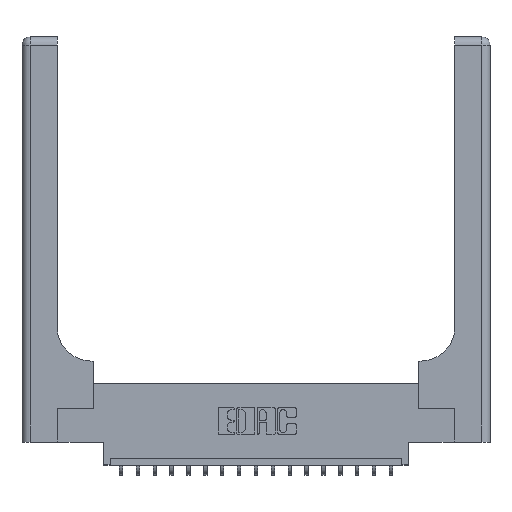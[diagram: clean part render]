
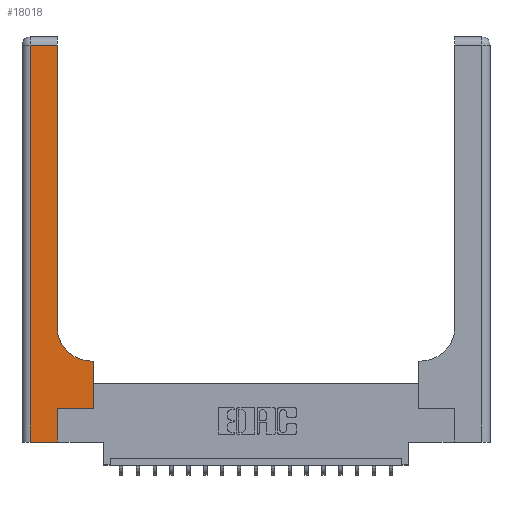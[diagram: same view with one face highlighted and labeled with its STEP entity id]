
A CAD part, top view. The second image highlights one B-rep face of the part: STEP entity #18018.
In plain terms, the highlighted planar face has unit normal (0, 0, 1).
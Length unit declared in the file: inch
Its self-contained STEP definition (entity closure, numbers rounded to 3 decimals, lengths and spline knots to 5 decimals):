
#52 = EDGE_CURVE ( 'NONE', #16930, #7713, #11292, .T. ) ;
#722 = EDGE_LOOP ( 'NONE', ( #4917, #16883, #13863, #2828, #6843, #11314, #15719, #741, #4698 ) ) ;
#741 = ORIENTED_EDGE ( 'NONE', *, *, #16131, .T. ) ;
#763 = VERTEX_POINT ( 'NONE', #7768 ) ;
#984 = DIRECTION ( 'NONE',  ( 1., 0., 0. ) ) ;
#1055 = EDGE_CURVE ( 'NONE', #16804, #16004, #9851, .T. ) ;
#1430 = VERTEX_POINT ( 'NONE', #13749 ) ;
#1799 = CARTESIAN_POINT ( 'NONE',  ( 0.26, 0.85, 0.37 ) ) ;
#2469 = CARTESIAN_POINT ( 'NONE',  ( 0.26, 2.94, 0.37 ) ) ;
#2828 = ORIENTED_EDGE ( 'NONE', *, *, #13575, .T. ) ;
#3823 = LINE ( 'NONE', #15802, #11369 ) ;
#4076 = DIRECTION ( 'NONE',  ( 0., 1., 0. ) ) ;
#4698 = ORIENTED_EDGE ( 'NONE', *, *, #8506, .T. ) ;
#4772 = PLANE ( 'NONE',  #10855 ) ;
#4830 = VERTEX_POINT ( 'NONE', #11650 ) ;
#4917 = ORIENTED_EDGE ( 'NONE', *, *, #7274, .T. ) ;
#5082 = VERTEX_POINT ( 'NONE', #1799 ) ;
#5216 = LINE ( 'NONE', #12580, #8334 ) ;
#5824 = VECTOR ( 'NONE', #984, 39.37008 ) ;
#5890 = VECTOR ( 'NONE', #4076, 39.37008 ) ;
#6302 = CARTESIAN_POINT ( 'NONE',  ( 0., 3., 0.37 ) ) ;
#6549 = CARTESIAN_POINT ( 'NONE',  ( 0.51, 0.85, 0.37 ) ) ;
#6659 = DIRECTION ( 'NONE',  ( -1., 0., 0. ) ) ;
#6843 = ORIENTED_EDGE ( 'NONE', *, *, #10674, .T. ) ;
#6967 = AXIS2_PLACEMENT_3D ( 'NONE', #6549, #16999, #8089 ) ;
#7274 = EDGE_CURVE ( 'NONE', #5082, #8728, #3823, .T. ) ;
#7713 = VERTEX_POINT ( 'NONE', #15285 ) ;
#7768 = CARTESIAN_POINT ( 'NONE',  ( 0.265, 0., 0.37 ) ) ;
#7836 = DIRECTION ( 'NONE',  ( 0., 0., -1. ) ) ;
#8089 = DIRECTION ( 'NONE',  ( 1., 0., 0. ) ) ;
#8334 = VECTOR ( 'NONE', #11222, 39.37008 ) ;
#8506 = EDGE_CURVE ( 'NONE', #1430, #5082, #15771, .T. ) ;
#8728 = VERTEX_POINT ( 'NONE', #2469 ) ;
#9010 = CARTESIAN_POINT ( 'NONE',  ( 0.528, 0.25, 0.37 ) ) ;
#9616 = FACE_OUTER_BOUND ( 'NONE', #722, .T. ) ;
#9851 = LINE ( 'NONE', #18771, #5824 ) ;
#10055 = DIRECTION ( 'NONE',  ( 1., 0., 0. ) ) ;
#10365 = VECTOR ( 'NONE', #19259, 39.37008 ) ;
#10436 = CARTESIAN_POINT ( 'NONE',  ( 0.06, 3., 0.37 ) ) ;
#10502 = DIRECTION ( 'NONE',  ( 0., 1., 0. ) ) ;
#10674 = EDGE_CURVE ( 'NONE', #763, #16804, #19159, .T. ) ;
#10782 = EDGE_CURVE ( 'NONE', #16004, #4830, #12474, .T. ) ;
#10855 = AXIS2_PLACEMENT_3D ( 'NONE', #6302, #7836, #18221 ) ;
#11222 = DIRECTION ( 'NONE',  ( -1., 0., 0. ) ) ;
#11264 = CARTESIAN_POINT ( 'NONE',  ( 0.265, 0.25, 0.37 ) ) ;
#11292 = LINE ( 'NONE', #10436, #10365 ) ;
#11314 = ORIENTED_EDGE ( 'NONE', *, *, #1055, .T. ) ;
#11369 = VECTOR ( 'NONE', #17298, 39.37008 ) ;
#11650 = CARTESIAN_POINT ( 'NONE',  ( 0.528, 0.6, 0.37 ) ) ;
#12358 = VECTOR ( 'NONE', #10055, 39.37008 ) ;
#12474 = LINE ( 'NONE', #9010, #15951 ) ;
#12580 = CARTESIAN_POINT ( 'NONE',  ( 0.26, 0.6, 0.37 ) ) ;
#13575 = EDGE_CURVE ( 'NONE', #7713, #763, #16302, .T. ) ;
#13690 = CARTESIAN_POINT ( 'NONE',  ( 0.528, 0.25, 0.37 ) ) ;
#13749 = CARTESIAN_POINT ( 'NONE',  ( 0.51, 0.6, 0.37 ) ) ;
#13863 = ORIENTED_EDGE ( 'NONE', *, *, #52, .T. ) ;
#14120 = EDGE_CURVE ( 'NONE', #8728, #16930, #18785, .T. ) ;
#14462 = CARTESIAN_POINT ( 'NONE',  ( 0., 0., 0.37 ) ) ;
#14596 = CARTESIAN_POINT ( 'NONE',  ( 0.265, 0., 0.37 ) ) ;
#14900 = VECTOR ( 'NONE', #6659, 39.37008 ) ;
#15285 = CARTESIAN_POINT ( 'NONE',  ( 0.06, 0., 0.37 ) ) ;
#15607 = CARTESIAN_POINT ( 'NONE',  ( 0., 2.94, 0.37 ) ) ;
#15719 = ORIENTED_EDGE ( 'NONE', *, *, #10782, .T. ) ;
#15771 = CIRCLE ( 'NONE', #6967, 0.25 ) ;
#15802 = CARTESIAN_POINT ( 'NONE',  ( 0.26, 3., 0.37 ) ) ;
#15951 = VECTOR ( 'NONE', #10502, 39.37008 ) ;
#15998 = CARTESIAN_POINT ( 'NONE',  ( 0.06, 2.94, 0.37 ) ) ;
#16004 = VERTEX_POINT ( 'NONE', #13690 ) ;
#16131 = EDGE_CURVE ( 'NONE', #4830, #1430, #5216, .T. ) ;
#16302 = LINE ( 'NONE', #14462, #12358 ) ;
#16804 = VERTEX_POINT ( 'NONE', #11264 ) ;
#16883 = ORIENTED_EDGE ( 'NONE', *, *, #14120, .T. ) ;
#16930 = VERTEX_POINT ( 'NONE', #15998 ) ;
#16999 = DIRECTION ( 'NONE',  ( 0., 0., -1. ) ) ;
#17298 = DIRECTION ( 'NONE',  ( 0., 1., 0. ) ) ;
#18018 = ADVANCED_FACE ( 'NONE', ( #9616 ), #4772, .F. ) ;
#18221 = DIRECTION ( 'NONE',  ( -1., 0., 0. ) ) ;
#18771 = CARTESIAN_POINT ( 'NONE',  ( 0.265, 0.25, 0.37 ) ) ;
#18785 = LINE ( 'NONE', #15607, #14900 ) ;
#19159 = LINE ( 'NONE', #14596, #5890 ) ;
#19259 = DIRECTION ( 'NONE',  ( 0., -1., 0. ) ) ;
